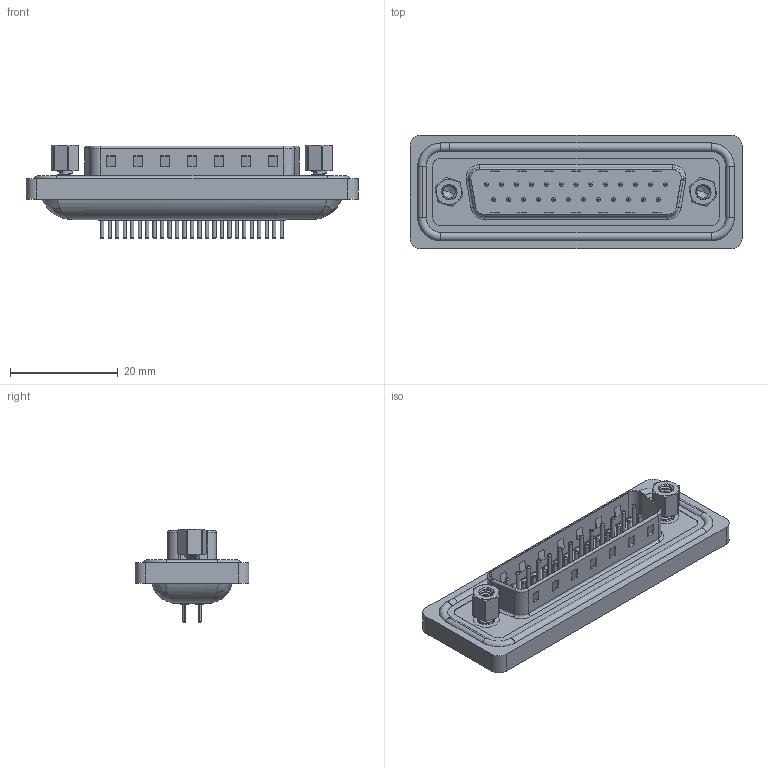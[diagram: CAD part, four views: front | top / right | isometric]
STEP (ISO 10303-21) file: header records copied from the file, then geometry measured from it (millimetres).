
FILE_DESCRIPTION (( 'STEP AP203' ), '1' );
FILE_NAME ('627-W25-220-012.STEP', '2024-03-19T12:00:55', ( '' ), ( '' ), 'SwSTEP 2.0', 'SolidWorks 2023', '' );
FILE_SCHEMA (( 'CONFIG_CONTROL_DESIGN' ));
Length unit declared in the file: millimetre
Products named in the file (8): 627W Shell Front_25 Contacts; 627W Contact Row 2_20; 627W Contact Row 1_20; 627W 4-40 Hex Standoff; 627W Housing_25 Contacts; 627-W25-220-012; 627W Waterproof Housing_25 Contacts; 627W 4-40 Threaded Rivet
Assembly tree (32 placements, depth 2):
  627-W25-220-012
    627W Housing_25 Contacts
    627W Shell Front_25 Contacts
    627W Contact Row 1_20  x13
    627W Contact Row 2_20  x12
    627W Waterproof Housing_25 Contacts
    627W 4-40 Threaded Rivet  x2
    627W 4-40 Hex Standoff  x2
Bounding box: 61.5 x 21.1 x 17.4 mm (x, y, z)
Volume: 7470.6 mm3; surface area: 11062.3 mm2
Topology: 33 solids, 33 shells, 1495 faces, 3352 edges, 2059 vertices
Faces by surface type: cylinder 620, torus 443, plane 380, cone 30, bspline 22
Entity records: 27760 total; most frequent: CARTESIAN_POINT 8209, DIRECTION 3983, ORIENTED_EDGE 3604, EDGE_CURVE 1802, AXIS2_PLACEMENT_3D 1572, VERTEX_POINT 1158, EDGE_LOOP 940, VECTOR 839
